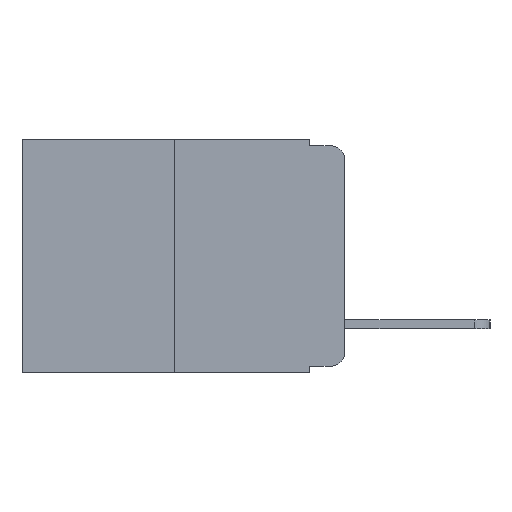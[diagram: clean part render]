
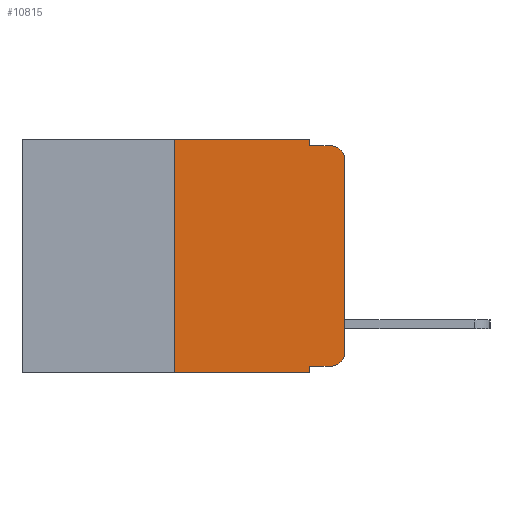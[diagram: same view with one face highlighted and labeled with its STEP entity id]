
A CAD part, left-side view. The second image highlights one B-rep face of the part: STEP entity #10815.
In plain terms, the highlighted planar face has unit normal (-1, 0, 0).
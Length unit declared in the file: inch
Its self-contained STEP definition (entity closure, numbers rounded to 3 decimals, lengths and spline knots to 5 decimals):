
#45 = CARTESIAN_POINT ( 'NONE',  ( 0., 0., -0.313 ) ) ;
#936 = PLANE ( 'NONE',  #23485 ) ;
#1177 = VECTOR ( 'NONE', #13939, 39.37008 ) ;
#1674 = VECTOR ( 'NONE', #8747, 39.37008 ) ;
#1970 = CARTESIAN_POINT ( 'NONE',  ( 0., 0.473, 0. ) ) ;
#1995 = VERTEX_POINT ( 'NONE', #16549 ) ;
#2178 = DIRECTION ( 'NONE',  ( 0., 0., -1. ) ) ;
#2371 = LINE ( 'NONE', #9459, #20364 ) ;
#3360 = CARTESIAN_POINT ( 'NONE',  ( 0., 0.051, -0.01 ) ) ;
#3484 = VECTOR ( 'NONE', #9508, 39.37008 ) ;
#4070 = LINE ( 'NONE', #13263, #3484 ) ;
#4433 = VECTOR ( 'NONE', #12172, 39.37008 ) ;
#4560 = VECTOR ( 'NONE', #5795, 39.37008 ) ;
#5135 = LINE ( 'NONE', #1970, #4560 ) ;
#5572 = EDGE_CURVE ( 'NONE', #10089, #1995, #2371, .T. ) ;
#5638 = EDGE_CURVE ( 'NONE', #9090, #12805, #19774, .T. ) ;
#5652 = CARTESIAN_POINT ( 'NONE',  ( 0., 0.473, -0.343 ) ) ;
#5673 = VECTOR ( 'NONE', #22518, 39.37008 ) ;
#5795 = DIRECTION ( 'NONE',  ( 0., -1., 0. ) ) ;
#5929 = EDGE_LOOP ( 'NONE', ( #12538, #17989, #7968, #6100, #16804, #16353, #16164, #19249, #15064, #11491 ) ) ;
#6100 = ORIENTED_EDGE ( 'NONE', *, *, #8798, .F. ) ;
#6291 = EDGE_CURVE ( 'NONE', #10215, #19771, #10593, .T. ) ;
#6591 = CARTESIAN_POINT ( 'NONE',  ( 0., 0., -0.03 ) ) ;
#6873 = CARTESIAN_POINT ( 'NONE',  ( 0., 0., 0. ) ) ;
#7968 = ORIENTED_EDGE ( 'NONE', *, *, #5638, .F. ) ;
#8435 = CIRCLE ( 'NONE', #14681, 0.02 ) ;
#8747 = DIRECTION ( 'NONE',  ( 0., 0., 1. ) ) ;
#8798 = EDGE_CURVE ( 'NONE', #15007, #9090, #4070, .T. ) ;
#9090 = VERTEX_POINT ( 'NONE', #3360 ) ;
#9113 = CARTESIAN_POINT ( 'NONE',  ( 0., 0.25, 0. ) ) ;
#9255 = EDGE_CURVE ( 'NONE', #1995, #9396, #8435, .T. ) ;
#9396 = VERTEX_POINT ( 'NONE', #45 ) ;
#9459 = CARTESIAN_POINT ( 'NONE',  ( 0., 0.051, -0.333 ) ) ;
#9493 = DIRECTION ( 'NONE',  ( -1., 0., 0. ) ) ;
#9508 = DIRECTION ( 'NONE',  ( 0., 0., -1. ) ) ;
#10089 = VERTEX_POINT ( 'NONE', #21122 ) ;
#10215 = VERTEX_POINT ( 'NONE', #15885 ) ;
#10379 = CARTESIAN_POINT ( 'NONE',  ( 0., 0.473, 0. ) ) ;
#10593 = LINE ( 'NONE', #5652, #5673 ) ;
#10815 = ADVANCED_FACE ( 'NONE', ( #10981 ), #936, .F. ) ;
#10945 = DIRECTION ( 'NONE',  ( -1., 0., 0. ) ) ;
#10981 = FACE_OUTER_BOUND ( 'NONE', #5929, .T. ) ;
#11164 = LINE ( 'NONE', #12106, #1177 ) ;
#11348 = CARTESIAN_POINT ( 'NONE',  ( 0., 0.02, -0.01 ) ) ;
#11491 = ORIENTED_EDGE ( 'NONE', *, *, #9255, .T. ) ;
#12106 = CARTESIAN_POINT ( 'NONE',  ( 0., 0.25, 0. ) ) ;
#12172 = DIRECTION ( 'NONE',  ( 0., -1., 0. ) ) ;
#12201 = LINE ( 'NONE', #6873, #1674 ) ;
#12224 = DIRECTION ( 'NONE',  ( 0., 0., -1. ) ) ;
#12538 = ORIENTED_EDGE ( 'NONE', *, *, #18942, .T. ) ;
#12805 = VERTEX_POINT ( 'NONE', #11348 ) ;
#13263 = CARTESIAN_POINT ( 'NONE',  ( 0., 0.051, 0. ) ) ;
#13939 = DIRECTION ( 'NONE',  ( 0., 0., 1. ) ) ;
#14068 = EDGE_CURVE ( 'NONE', #17785, #15007, #5135, .T. ) ;
#14494 = CIRCLE ( 'NONE', #14647, 0.02 ) ;
#14647 = AXIS2_PLACEMENT_3D ( 'NONE', #20517, #9493, #22337 ) ;
#14681 = AXIS2_PLACEMENT_3D ( 'NONE', #21940, #10945, #23777 ) ;
#15007 = VERTEX_POINT ( 'NONE', #22902 ) ;
#15064 = ORIENTED_EDGE ( 'NONE', *, *, #5572, .T. ) ;
#15148 = CARTESIAN_POINT ( 'NONE',  ( 0., 0.051, 0. ) ) ;
#15642 = EDGE_CURVE ( 'NONE', #10215, #17785, #11164, .T. ) ;
#15885 = CARTESIAN_POINT ( 'NONE',  ( 0., 0.25, -0.343 ) ) ;
#16164 = ORIENTED_EDGE ( 'NONE', *, *, #6291, .T. ) ;
#16353 = ORIENTED_EDGE ( 'NONE', *, *, #15642, .F. ) ;
#16549 = CARTESIAN_POINT ( 'NONE',  ( 0., 0.02, -0.333 ) ) ;
#16804 = ORIENTED_EDGE ( 'NONE', *, *, #14068, .F. ) ;
#16887 = VERTEX_POINT ( 'NONE', #6591 ) ;
#17203 = EDGE_CURVE ( 'NONE', #16887, #12805, #14494, .T. ) ;
#17280 = EDGE_CURVE ( 'NONE', #10089, #19771, #18273, .T. ) ;
#17785 = VERTEX_POINT ( 'NONE', #9113 ) ;
#17989 = ORIENTED_EDGE ( 'NONE', *, *, #17203, .T. ) ;
#18273 = LINE ( 'NONE', #15148, #21991 ) ;
#18942 = EDGE_CURVE ( 'NONE', #9396, #16887, #12201, .T. ) ;
#19249 = ORIENTED_EDGE ( 'NONE', *, *, #17280, .F. ) ;
#19771 = VERTEX_POINT ( 'NONE', #22194 ) ;
#19774 = LINE ( 'NONE', #20384, #4433 ) ;
#20364 = VECTOR ( 'NONE', #21855, 39.37008 ) ;
#20384 = CARTESIAN_POINT ( 'NONE',  ( 0., 0.051, -0.01 ) ) ;
#20517 = CARTESIAN_POINT ( 'NONE',  ( 0., 0.02, -0.03 ) ) ;
#21122 = CARTESIAN_POINT ( 'NONE',  ( 0., 0.051, -0.333 ) ) ;
#21855 = DIRECTION ( 'NONE',  ( 0., -1., 0. ) ) ;
#21940 = CARTESIAN_POINT ( 'NONE',  ( 0., 0.02, -0.313 ) ) ;
#21991 = VECTOR ( 'NONE', #2178, 39.37008 ) ;
#22194 = CARTESIAN_POINT ( 'NONE',  ( 0., 0.051, -0.343 ) ) ;
#22337 = DIRECTION ( 'NONE',  ( 0., 0., -1. ) ) ;
#22518 = DIRECTION ( 'NONE',  ( 0., -1., 0. ) ) ;
#22902 = CARTESIAN_POINT ( 'NONE',  ( 0., 0.051, 0. ) ) ;
#23221 = DIRECTION ( 'NONE',  ( 1., 0., 0. ) ) ;
#23485 = AXIS2_PLACEMENT_3D ( 'NONE', #10379, #23221, #12224 ) ;
#23777 = DIRECTION ( 'NONE',  ( 0., 0., -1. ) ) ;
